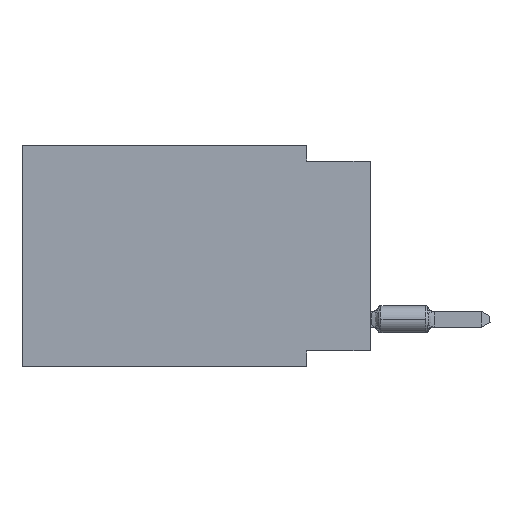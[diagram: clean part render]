
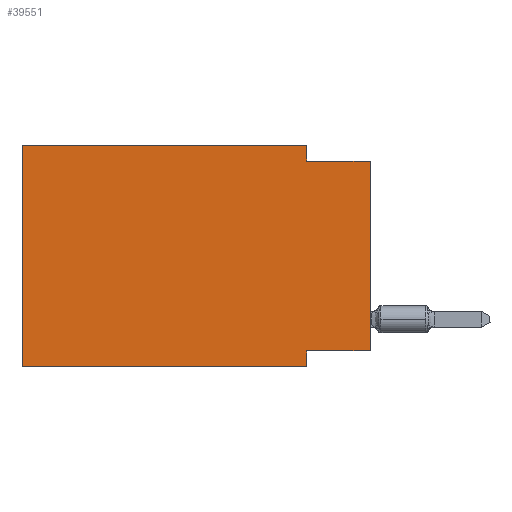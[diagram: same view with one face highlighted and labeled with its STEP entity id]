
A CAD part, left-side view. The second image highlights one B-rep face of the part: STEP entity #39551.
In plain terms, the highlighted planar face has unit normal (-1, 0, 0).
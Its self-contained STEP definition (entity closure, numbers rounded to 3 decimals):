
#292 = DIRECTION ( 'NONE',  ( 0., -1., 0. ) ) ;
#2151 = LINE ( 'NONE', #21592, #25539 ) ;
#3728 = CARTESIAN_POINT ( 'NONE',  ( 0., 13.97, 0. ) ) ;
#4895 = VERTEX_POINT ( 'NONE', #55481 ) ;
#6513 = VERTEX_POINT ( 'NONE', #52768 ) ;
#6596 = AXIS2_PLACEMENT_3D ( 'NONE', #37980, #22742, #61546 ) ;
#6814 = VERTEX_POINT ( 'NONE', #45720 ) ;
#8992 = EDGE_LOOP ( 'NONE', ( #41423, #18388, #36840, #21527, #10351, #30689, #53155, #59788 ) ) ;
#9123 = VECTOR ( 'NONE', #58358, 1000. ) ;
#10351 = ORIENTED_EDGE ( 'NONE', *, *, #28796, .F. ) ;
#12267 = VERTEX_POINT ( 'NONE', #62777 ) ;
#12966 = CARTESIAN_POINT ( 'NONE',  ( 0., 2.54, 0. ) ) ;
#14080 = CARTESIAN_POINT ( 'NONE',  ( 0., 0., -0.635 ) ) ;
#16524 = LINE ( 'NONE', #21271, #36776 ) ;
#17118 = DIRECTION ( 'NONE',  ( 0., 1., 0. ) ) ;
#17438 = DIRECTION ( 'NONE',  ( 0., 0., 1. ) ) ;
#18388 = ORIENTED_EDGE ( 'NONE', *, *, #47423, .F. ) ;
#18530 = CARTESIAN_POINT ( 'NONE',  ( 0., 0., 0. ) ) ;
#18832 = VECTOR ( 'NONE', #28351, 1000. ) ;
#19128 = LINE ( 'NONE', #18530, #18832 ) ;
#19473 = CARTESIAN_POINT ( 'NONE',  ( 0., 2.54, 0. ) ) ;
#20043 = VERTEX_POINT ( 'NONE', #58160 ) ;
#21271 = CARTESIAN_POINT ( 'NONE',  ( 0., 0., -8.255 ) ) ;
#21527 = ORIENTED_EDGE ( 'NONE', *, *, #28498, .F. ) ;
#21592 = CARTESIAN_POINT ( 'NONE',  ( 0., 2.54, -8.89 ) ) ;
#22206 = VERTEX_POINT ( 'NONE', #12966 ) ;
#22340 = VECTOR ( 'NONE', #292, 1000. ) ;
#22742 = DIRECTION ( 'NONE',  ( 1., 0., 0. ) ) ;
#22757 = VERTEX_POINT ( 'NONE', #52955 ) ;
#24067 = VECTOR ( 'NONE', #54123, 1000. ) ;
#24442 = VECTOR ( 'NONE', #17438, 1000. ) ;
#25539 = VECTOR ( 'NONE', #54633, 1000. ) ;
#27487 = FACE_OUTER_BOUND ( 'NONE', #8992, .T. ) ;
#28001 = CARTESIAN_POINT ( 'NONE',  ( 0., 0., -0.635 ) ) ;
#28351 = DIRECTION ( 'NONE',  ( 0., 0., 1. ) ) ;
#28498 = EDGE_CURVE ( 'NONE', #6814, #22206, #43860, .T. ) ;
#28796 = EDGE_CURVE ( 'NONE', #4895, #6814, #32065, .T. ) ;
#30210 = EDGE_CURVE ( 'NONE', #6513, #20043, #16524, .T. ) ;
#30689 = ORIENTED_EDGE ( 'NONE', *, *, #51934, .T. ) ;
#32065 = LINE ( 'NONE', #3728, #24442 ) ;
#36776 = VECTOR ( 'NONE', #17118, 1000. ) ;
#36840 = ORIENTED_EDGE ( 'NONE', *, *, #62062, .F. ) ;
#37980 = CARTESIAN_POINT ( 'NONE',  ( 0., 13.97, 0. ) ) ;
#38849 = DIRECTION ( 'NONE',  ( 0., 0., -1. ) ) ;
#39551 = ADVANCED_FACE ( 'NONE', ( #27487 ), #61861, .F. ) ;
#40039 = EDGE_CURVE ( 'NONE', #6513, #45930, #19128, .T. ) ;
#41423 = ORIENTED_EDGE ( 'NONE', *, *, #40039, .T. ) ;
#43860 = LINE ( 'NONE', #57862, #22340 ) ;
#45720 = CARTESIAN_POINT ( 'NONE',  ( 0., 13.97, 0. ) ) ;
#45930 = VERTEX_POINT ( 'NONE', #28001 ) ;
#46587 = LINE ( 'NONE', #61254, #9123 ) ;
#47423 = EDGE_CURVE ( 'NONE', #12267, #45930, #58871, .T. ) ;
#51934 = EDGE_CURVE ( 'NONE', #4895, #22757, #46587, .T. ) ;
#52768 = CARTESIAN_POINT ( 'NONE',  ( 0., 0., -8.255 ) ) ;
#52955 = CARTESIAN_POINT ( 'NONE',  ( 0., 2.54, -8.89 ) ) ;
#53155 = ORIENTED_EDGE ( 'NONE', *, *, #54775, .F. ) ;
#54123 = DIRECTION ( 'NONE',  ( 0., -1., 0. ) ) ;
#54633 = DIRECTION ( 'NONE',  ( 0., 0., -1. ) ) ;
#54775 = EDGE_CURVE ( 'NONE', #20043, #22757, #2151, .T. ) ;
#54952 = LINE ( 'NONE', #19473, #61681 ) ;
#55481 = CARTESIAN_POINT ( 'NONE',  ( 0., 13.97, -8.89 ) ) ;
#57862 = CARTESIAN_POINT ( 'NONE',  ( 0., 13.97, 0. ) ) ;
#58160 = CARTESIAN_POINT ( 'NONE',  ( 0., 2.54, -8.255 ) ) ;
#58358 = DIRECTION ( 'NONE',  ( 0., -1., 0. ) ) ;
#58871 = LINE ( 'NONE', #14080, #24067 ) ;
#59788 = ORIENTED_EDGE ( 'NONE', *, *, #30210, .F. ) ;
#61254 = CARTESIAN_POINT ( 'NONE',  ( 0., 13.97, -8.89 ) ) ;
#61546 = DIRECTION ( 'NONE',  ( 0., 0., -1. ) ) ;
#61681 = VECTOR ( 'NONE', #38849, 1000. ) ;
#61861 = PLANE ( 'NONE',  #6596 ) ;
#62062 = EDGE_CURVE ( 'NONE', #22206, #12267, #54952, .T. ) ;
#62777 = CARTESIAN_POINT ( 'NONE',  ( 0., 2.54, -0.635 ) ) ;
